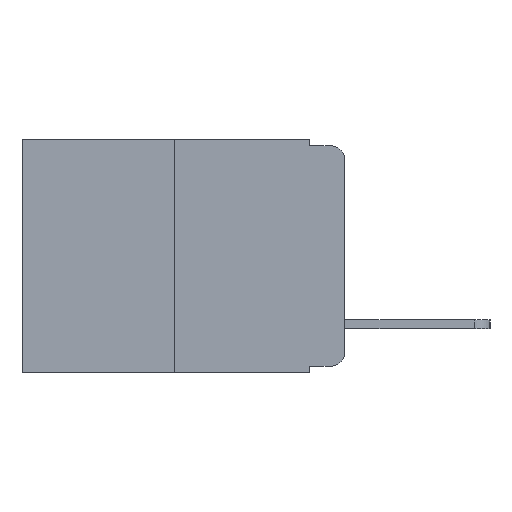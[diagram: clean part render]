
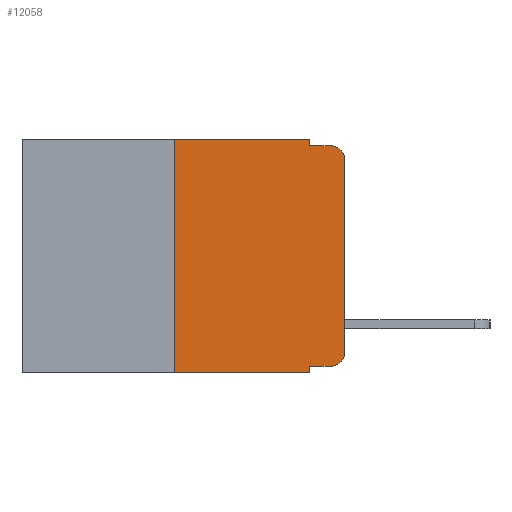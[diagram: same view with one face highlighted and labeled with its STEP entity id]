
A CAD part, left-side view. The second image highlights one B-rep face of the part: STEP entity #12058.
In plain terms, the highlighted planar face has unit normal (-1, 0, 0).
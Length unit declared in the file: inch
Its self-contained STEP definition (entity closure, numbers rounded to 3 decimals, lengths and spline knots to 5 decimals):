
#133 = ORIENTED_EDGE ( 'NONE', *, *, #10697, .F. ) ;
#1885 = PLANE ( 'NONE',  #14493 ) ;
#2091 = VECTOR ( 'NONE', #21684, 39.37008 ) ;
#2573 = AXIS2_PLACEMENT_3D ( 'NONE', #3405, #16621, #5360 ) ;
#2695 = VERTEX_POINT ( 'NONE', #7885 ) ;
#2787 = LINE ( 'NONE', #18499, #21622 ) ;
#3035 = LINE ( 'NONE', #4276, #12577 ) ;
#3311 = EDGE_CURVE ( 'NONE', #8052, #22807, #22744, .T. ) ;
#3405 = CARTESIAN_POINT ( 'NONE',  ( 0., 0.02, -0.313 ) ) ;
#3936 = CARTESIAN_POINT ( 'NONE',  ( 0., 0.051, -0.333 ) ) ;
#4016 = FACE_OUTER_BOUND ( 'NONE', #21788, .T. ) ;
#4147 = ORIENTED_EDGE ( 'NONE', *, *, #16919, .T. ) ;
#4276 = CARTESIAN_POINT ( 'NONE',  ( 0., 0., 0. ) ) ;
#4296 = EDGE_CURVE ( 'NONE', #10209, #23299, #19717, .T. ) ;
#4761 = CARTESIAN_POINT ( 'NONE',  ( 0., 0.051, -0.333 ) ) ;
#4923 = LINE ( 'NONE', #21911, #24228 ) ;
#5360 = DIRECTION ( 'NONE',  ( 0., 0., -1. ) ) ;
#5598 = EDGE_CURVE ( 'NONE', #16804, #10209, #14193, .T. ) ;
#5791 = CARTESIAN_POINT ( 'NONE',  ( 0., 0.02, -0.03 ) ) ;
#5821 = DIRECTION ( 'NONE',  ( 0., 0., -1. ) ) ;
#5959 = CARTESIAN_POINT ( 'NONE',  ( 0., 0.051, -0.01 ) ) ;
#5973 = ORIENTED_EDGE ( 'NONE', *, *, #12568, .F. ) ;
#6227 = DIRECTION ( 'NONE',  ( 0., 0., 1. ) ) ;
#6486 = AXIS2_PLACEMENT_3D ( 'NONE', #5791, #18874, #7734 ) ;
#6575 = ORIENTED_EDGE ( 'NONE', *, *, #3311, .T. ) ;
#7379 = LINE ( 'NONE', #10428, #15030 ) ;
#7734 = DIRECTION ( 'NONE',  ( 0., 0., -1. ) ) ;
#7781 = ORIENTED_EDGE ( 'NONE', *, *, #4296, .T. ) ;
#7885 = CARTESIAN_POINT ( 'NONE',  ( 0., 0.051, 0. ) ) ;
#8052 = VERTEX_POINT ( 'NONE', #21762 ) ;
#8176 = EDGE_CURVE ( 'NONE', #16804, #22807, #2787, .T. ) ;
#9261 = DIRECTION ( 'NONE',  ( 0., 0., -1. ) ) ;
#9454 = EDGE_CURVE ( 'NONE', #8052, #15838, #22720, .T. ) ;
#10209 = VERTEX_POINT ( 'NONE', #20057 ) ;
#10428 = CARTESIAN_POINT ( 'NONE',  ( 0., 0.051, 0. ) ) ;
#10697 = EDGE_CURVE ( 'NONE', #2695, #14516, #7379, .T. ) ;
#10921 = DIRECTION ( 'NONE',  ( 0., -1., 0. ) ) ;
#11024 = ORIENTED_EDGE ( 'NONE', *, *, #9454, .F. ) ;
#11466 = CARTESIAN_POINT ( 'NONE',  ( 0., 0., -0.03 ) ) ;
#11517 = CARTESIAN_POINT ( 'NONE',  ( 0., 0.051, -0.343 ) ) ;
#11731 = VECTOR ( 'NONE', #10921, 39.37008 ) ;
#12058 = ADVANCED_FACE ( 'NONE', ( #4016 ), #1885, .F. ) ;
#12173 = ORIENTED_EDGE ( 'NONE', *, *, #5598, .T. ) ;
#12568 = EDGE_CURVE ( 'NONE', #15838, #2695, #22179, .T. ) ;
#12577 = VECTOR ( 'NONE', #6227, 39.37008 ) ;
#13196 = EDGE_CURVE ( 'NONE', #14516, #24361, #4923, .T. ) ;
#14193 = LINE ( 'NONE', #4761, #18500 ) ;
#14229 = ORIENTED_EDGE ( 'NONE', *, *, #14464, .T. ) ;
#14464 = EDGE_CURVE ( 'NONE', #15710, #24361, #21294, .T. ) ;
#14493 = AXIS2_PLACEMENT_3D ( 'NONE', #15147, #17051, #5821 ) ;
#14516 = VERTEX_POINT ( 'NONE', #5959 ) ;
#14589 = CARTESIAN_POINT ( 'NONE',  ( 0., 0.473, 0. ) ) ;
#15030 = VECTOR ( 'NONE', #17800, 39.37008 ) ;
#15147 = CARTESIAN_POINT ( 'NONE',  ( 0., 0.473, 0. ) ) ;
#15710 = VERTEX_POINT ( 'NONE', #11466 ) ;
#15838 = VERTEX_POINT ( 'NONE', #21100 ) ;
#16548 = ORIENTED_EDGE ( 'NONE', *, *, #8176, .F. ) ;
#16621 = DIRECTION ( 'NONE',  ( -1., 0., 0. ) ) ;
#16804 = VERTEX_POINT ( 'NONE', #3936 ) ;
#16919 = EDGE_CURVE ( 'NONE', #23299, #15710, #3035, .T. ) ;
#17051 = DIRECTION ( 'NONE',  ( 1., 0., 0. ) ) ;
#17094 = CARTESIAN_POINT ( 'NONE',  ( 0., 0., -0.313 ) ) ;
#17556 = CARTESIAN_POINT ( 'NONE',  ( 0., 0.473, -0.343 ) ) ;
#17800 = DIRECTION ( 'NONE',  ( 0., 0., -1. ) ) ;
#17802 = VECTOR ( 'NONE', #19381, 39.37008 ) ;
#18024 = CARTESIAN_POINT ( 'NONE',  ( 0., 0.25, 0. ) ) ;
#18255 = DIRECTION ( 'NONE',  ( 0., -1., 0. ) ) ;
#18499 = CARTESIAN_POINT ( 'NONE',  ( 0., 0.051, 0. ) ) ;
#18500 = VECTOR ( 'NONE', #19809, 39.37008 ) ;
#18874 = DIRECTION ( 'NONE',  ( -1., 0., 0. ) ) ;
#19381 = DIRECTION ( 'NONE',  ( 0., -1., 0. ) ) ;
#19717 = CIRCLE ( 'NONE', #2573, 0.02 ) ;
#19809 = DIRECTION ( 'NONE',  ( 0., -1., 0. ) ) ;
#20057 = CARTESIAN_POINT ( 'NONE',  ( 0., 0.02, -0.333 ) ) ;
#21100 = CARTESIAN_POINT ( 'NONE',  ( 0., 0.25, 0. ) ) ;
#21294 = CIRCLE ( 'NONE', #6486, 0.02 ) ;
#21622 = VECTOR ( 'NONE', #9261, 39.37008 ) ;
#21684 = DIRECTION ( 'NONE',  ( 0., 0., 1. ) ) ;
#21762 = CARTESIAN_POINT ( 'NONE',  ( 0., 0.25, -0.343 ) ) ;
#21788 = EDGE_LOOP ( 'NONE', ( #4147, #14229, #24052, #133, #5973, #11024, #6575, #16548, #12173, #7781 ) ) ;
#21911 = CARTESIAN_POINT ( 'NONE',  ( 0., 0.051, -0.01 ) ) ;
#22179 = LINE ( 'NONE', #14589, #11731 ) ;
#22720 = LINE ( 'NONE', #18024, #2091 ) ;
#22744 = LINE ( 'NONE', #17556, #17802 ) ;
#22807 = VERTEX_POINT ( 'NONE', #11517 ) ;
#23299 = VERTEX_POINT ( 'NONE', #17094 ) ;
#23831 = CARTESIAN_POINT ( 'NONE',  ( 0., 0.02, -0.01 ) ) ;
#24052 = ORIENTED_EDGE ( 'NONE', *, *, #13196, .F. ) ;
#24228 = VECTOR ( 'NONE', #18255, 39.37008 ) ;
#24361 = VERTEX_POINT ( 'NONE', #23831 ) ;
